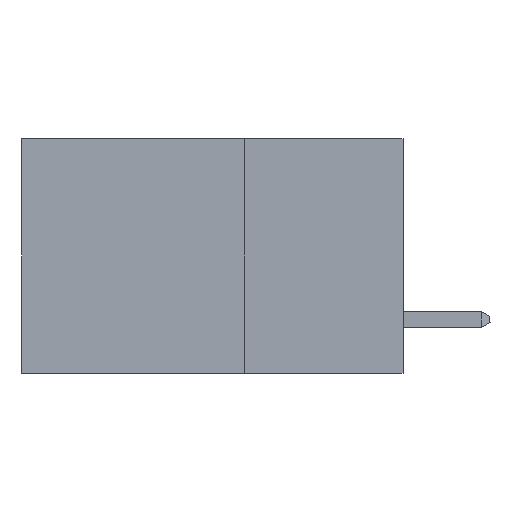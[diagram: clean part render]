
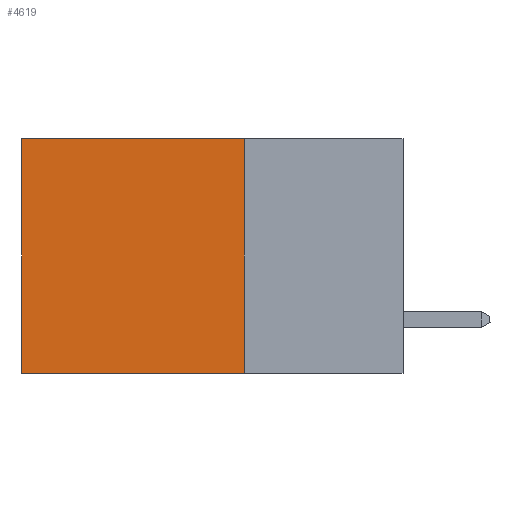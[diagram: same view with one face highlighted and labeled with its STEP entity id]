
A CAD part, left-side view. The second image highlights one B-rep face of the part: STEP entity #4619.
In plain terms, the highlighted planar face has unit normal (-1, 0, 0).
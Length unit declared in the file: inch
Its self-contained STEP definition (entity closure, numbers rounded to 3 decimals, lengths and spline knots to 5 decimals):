
#578 = CARTESIAN_POINT ( 'NONE',  ( 0.2875, 0.25, 0. ) ) ;
#833 = CARTESIAN_POINT ( 'NONE',  ( 0.2875, 0.25, -0.37 ) ) ;
#1643 = FACE_OUTER_BOUND ( 'NONE', #21364, .T. ) ;
#1825 = VECTOR ( 'NONE', #11842, 39.37008 ) ;
#2083 = VERTEX_POINT ( 'NONE', #578 ) ;
#2403 = ORIENTED_EDGE ( 'NONE', *, *, #13306, .F. ) ;
#2967 = CARTESIAN_POINT ( 'NONE',  ( 0.2875, 0.25, 0. ) ) ;
#4619 = ADVANCED_FACE ( 'NONE', ( #1643 ), #9803, .F. ) ;
#4960 = CARTESIAN_POINT ( 'NONE',  ( 0.2875, 0.6, -0.37 ) ) ;
#5661 = CARTESIAN_POINT ( 'NONE',  ( 0.2875, 0.25, -0.37 ) ) ;
#6428 = CARTESIAN_POINT ( 'NONE',  ( 0.2875, 0.6, 0. ) ) ;
#6990 = VERTEX_POINT ( 'NONE', #4960 ) ;
#7746 = VECTOR ( 'NONE', #12660, 39.37008 ) ;
#8321 = VECTOR ( 'NONE', #19696, 39.37008 ) ;
#9803 = PLANE ( 'NONE',  #11896 ) ;
#9993 = EDGE_CURVE ( 'NONE', #10641, #6990, #11649, .T. ) ;
#10640 = LINE ( 'NONE', #5661, #7746 ) ;
#10641 = VERTEX_POINT ( 'NONE', #6428 ) ;
#10723 = ORIENTED_EDGE ( 'NONE', *, *, #16208, .T. ) ;
#10749 = LINE ( 'NONE', #20123, #1825 ) ;
#11461 = DIRECTION ( 'NONE',  ( 0., 0., -1. ) ) ;
#11649 = LINE ( 'NONE', #16163, #19022 ) ;
#11842 = DIRECTION ( 'NONE',  ( 0., 1., 0. ) ) ;
#11896 = AXIS2_PLACEMENT_3D ( 'NONE', #2967, #19620, #11461 ) ;
#12660 = DIRECTION ( 'NONE',  ( 0., 1., 0. ) ) ;
#12861 = DIRECTION ( 'NONE',  ( 0., 0., -1. ) ) ;
#13306 = EDGE_CURVE ( 'NONE', #2083, #18811, #18557, .T. ) ;
#16163 = CARTESIAN_POINT ( 'NONE',  ( 0.2875, 0.6, 0. ) ) ;
#16208 = EDGE_CURVE ( 'NONE', #2083, #10641, #10749, .T. ) ;
#16470 = CARTESIAN_POINT ( 'NONE',  ( 0.2875, 0.25, 0. ) ) ;
#17033 = ORIENTED_EDGE ( 'NONE', *, *, #9993, .T. ) ;
#18270 = EDGE_CURVE ( 'NONE', #18811, #6990, #10640, .T. ) ;
#18557 = LINE ( 'NONE', #16470, #8321 ) ;
#18811 = VERTEX_POINT ( 'NONE', #833 ) ;
#19022 = VECTOR ( 'NONE', #12861, 39.37008 ) ;
#19620 = DIRECTION ( 'NONE',  ( 1., 0., 0. ) ) ;
#19696 = DIRECTION ( 'NONE',  ( 0., 0., -1. ) ) ;
#20065 = ORIENTED_EDGE ( 'NONE', *, *, #18270, .F. ) ;
#20123 = CARTESIAN_POINT ( 'NONE',  ( 0.2875, 0.25, 0. ) ) ;
#21364 = EDGE_LOOP ( 'NONE', ( #17033, #20065, #2403, #10723 ) ) ;
